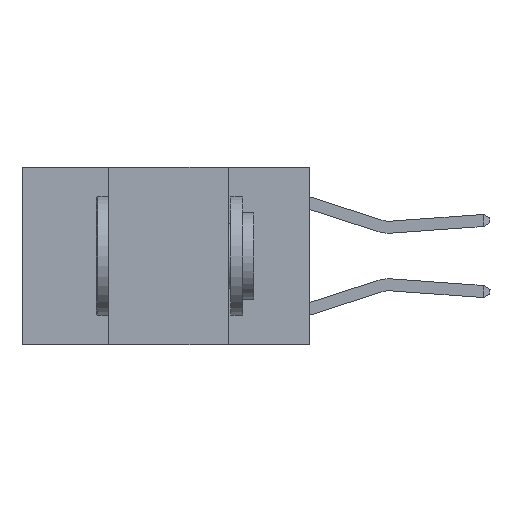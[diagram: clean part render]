
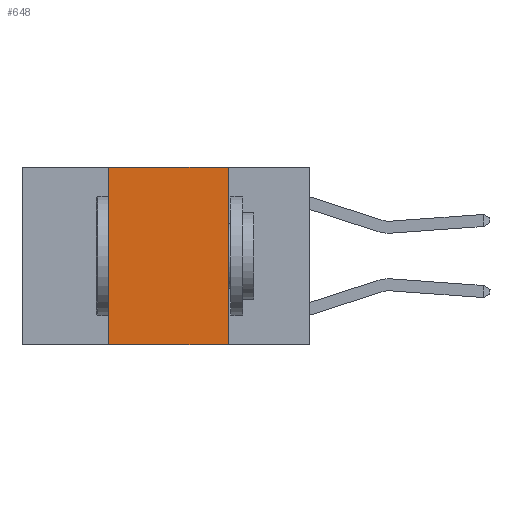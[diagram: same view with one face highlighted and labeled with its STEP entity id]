
A CAD part, left-side view. The second image highlights one B-rep face of the part: STEP entity #648.
In plain terms, the highlighted planar face has unit normal (-1, 0, 0).
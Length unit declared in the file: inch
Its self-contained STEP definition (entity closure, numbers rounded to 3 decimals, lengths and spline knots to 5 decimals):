
#131 = PLANE ( 'NONE',  #29475 ) ;
#552 = ORIENTED_EDGE ( 'NONE', *, *, #22275, .F. ) ;
#634 = VECTOR ( 'NONE', #9179, 39.37008 ) ;
#648 = ADVANCED_FACE ( 'NONE', ( #1162 ), #131, .F. ) ;
#1162 = FACE_OUTER_BOUND ( 'NONE', #17315, .T. ) ;
#1977 = CARTESIAN_POINT ( 'NONE',  ( 0., 0.42, 0. ) ) ;
#2138 = ORIENTED_EDGE ( 'NONE', *, *, #7546, .F. ) ;
#3600 = EDGE_CURVE ( 'NONE', #20387, #30970, #13987, .T. ) ;
#4109 = ORIENTED_EDGE ( 'NONE', *, *, #3600, .F. ) ;
#4193 = EDGE_CURVE ( 'NONE', #24051, #30970, #15093, .T. ) ;
#5228 = CARTESIAN_POINT ( 'NONE',  ( 0., 0.6, 0. ) ) ;
#6571 = CARTESIAN_POINT ( 'NONE',  ( 0., 0.17, 0. ) ) ;
#7032 = DIRECTION ( 'NONE',  ( 0., 0., 1. ) ) ;
#7546 = EDGE_CURVE ( 'NONE', #24051, #27358, #31359, .T. ) ;
#7732 = DIRECTION ( 'NONE',  ( 0., 0., -1. ) ) ;
#8462 = VECTOR ( 'NONE', #23593, 39.37008 ) ;
#8828 = ORIENTED_EDGE ( 'NONE', *, *, #4193, .T. ) ;
#8839 = CARTESIAN_POINT ( 'NONE',  ( 0., 0.6, -0.37 ) ) ;
#9179 = DIRECTION ( 'NONE',  ( 0., 0., -1. ) ) ;
#10533 = CARTESIAN_POINT ( 'NONE',  ( 0., 0.42, -0.37 ) ) ;
#11894 = VECTOR ( 'NONE', #7032, 39.37008 ) ;
#13987 = LINE ( 'NONE', #20831, #634 ) ;
#15093 = LINE ( 'NONE', #8839, #8462 ) ;
#16472 = CARTESIAN_POINT ( 'NONE',  ( 0., 0.6, 0. ) ) ;
#17315 = EDGE_LOOP ( 'NONE', ( #4109, #552, #2138, #8828 ) ) ;
#18910 = DIRECTION ( 'NONE',  ( 0., -1., 0. ) ) ;
#20387 = VERTEX_POINT ( 'NONE', #6571 ) ;
#20632 = LINE ( 'NONE', #16472, #25596 ) ;
#20831 = CARTESIAN_POINT ( 'NONE',  ( 0., 0.17, 0. ) ) ;
#22275 = EDGE_CURVE ( 'NONE', #27358, #20387, #20632, .T. ) ;
#22496 = DIRECTION ( 'NONE',  ( 1., 0., 0. ) ) ;
#23593 = DIRECTION ( 'NONE',  ( 0., -1., 0. ) ) ;
#24051 = VERTEX_POINT ( 'NONE', #10533 ) ;
#25596 = VECTOR ( 'NONE', #18910, 39.37008 ) ;
#26444 = CARTESIAN_POINT ( 'NONE',  ( 0., 0.42, 0. ) ) ;
#27358 = VERTEX_POINT ( 'NONE', #26444 ) ;
#29475 = AXIS2_PLACEMENT_3D ( 'NONE', #5228, #22496, #7732 ) ;
#29674 = CARTESIAN_POINT ( 'NONE',  ( 0., 0.17, -0.37 ) ) ;
#30970 = VERTEX_POINT ( 'NONE', #29674 ) ;
#31359 = LINE ( 'NONE', #1977, #11894 ) ;
